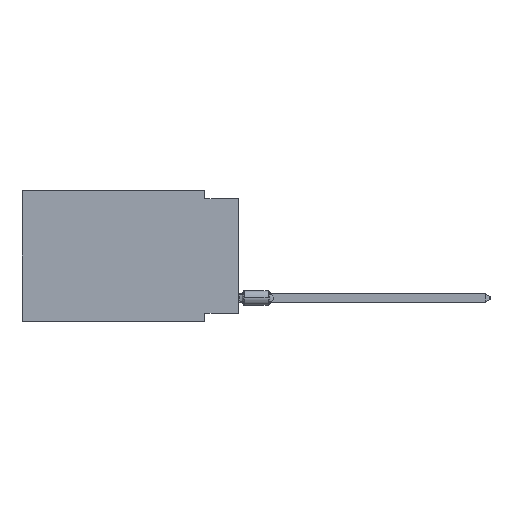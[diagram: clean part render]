
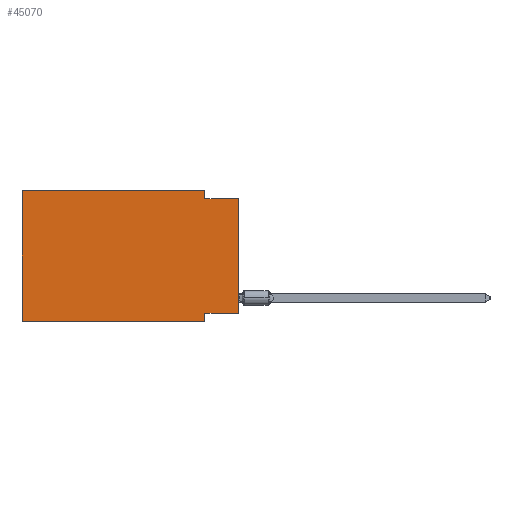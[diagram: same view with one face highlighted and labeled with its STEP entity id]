
A CAD part, left-side view. The second image highlights one B-rep face of the part: STEP entity #45070.
In plain terms, the highlighted planar face has unit normal (-1, 0, 0).
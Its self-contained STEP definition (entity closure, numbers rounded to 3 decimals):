
#275 = DIRECTION ( 'NONE',  ( 0., 0., -1. ) ) ;
#605 = DIRECTION ( 'NONE',  ( 1., 0., 0. ) ) ;
#1259 = DIRECTION ( 'NONE',  ( 0., 0., 1. ) ) ;
#1913 = VERTEX_POINT ( 'NONE', #60325 ) ;
#2238 = EDGE_CURVE ( 'NONE', #56575, #24521, #60573, .T. ) ;
#4235 = LINE ( 'NONE', #50794, #6742 ) ;
#4477 = ORIENTED_EDGE ( 'NONE', *, *, #44353, .F. ) ;
#4780 = VECTOR ( 'NONE', #49890, 1000. ) ;
#6014 = VERTEX_POINT ( 'NONE', #52594 ) ;
#6742 = VECTOR ( 'NONE', #49794, 1000. ) ;
#8410 = CARTESIAN_POINT ( 'NONE',  ( 0., 2.54, -9.906 ) ) ;
#9024 = LINE ( 'NONE', #14387, #4780 ) ;
#10152 = DIRECTION ( 'NONE',  ( 0., 0., -1. ) ) ;
#10315 = PLANE ( 'NONE',  #17072 ) ;
#10420 = EDGE_CURVE ( 'NONE', #21178, #6014, #4235, .T. ) ;
#11224 = VECTOR ( 'NONE', #1259, 1000. ) ;
#11340 = EDGE_CURVE ( 'NONE', #56575, #1913, #37415, .T. ) ;
#12109 = CARTESIAN_POINT ( 'NONE',  ( 0., 16.383, 0. ) ) ;
#12765 = LINE ( 'NONE', #12109, #43569 ) ;
#13588 = VECTOR ( 'NONE', #28830, 1000. ) ;
#14387 = CARTESIAN_POINT ( 'NONE',  ( 0., 16.383, 0. ) ) ;
#15198 = EDGE_CURVE ( 'NONE', #52797, #41607, #12765, .T. ) ;
#15515 = VECTOR ( 'NONE', #45199, 1000. ) ;
#15630 = CARTESIAN_POINT ( 'NONE',  ( 0., 0., -0.635 ) ) ;
#17072 = AXIS2_PLACEMENT_3D ( 'NONE', #35448, #605, #275 ) ;
#17195 = CARTESIAN_POINT ( 'NONE',  ( 0., 2.54, -0.635 ) ) ;
#17649 = CARTESIAN_POINT ( 'NONE',  ( 0., 0., 0. ) ) ;
#18766 = CARTESIAN_POINT ( 'NONE',  ( 0., 16.383, -9.906 ) ) ;
#21178 = VERTEX_POINT ( 'NONE', #18766 ) ;
#23139 = DIRECTION ( 'NONE',  ( 0., -1., 0. ) ) ;
#24521 = VERTEX_POINT ( 'NONE', #55439 ) ;
#24761 = CARTESIAN_POINT ( 'NONE',  ( 0., 0., -9.271 ) ) ;
#26007 = DIRECTION ( 'NONE',  ( 0., -1., 0. ) ) ;
#27126 = VERTEX_POINT ( 'NONE', #17195 ) ;
#28830 = DIRECTION ( 'NONE',  ( 0., 0., -1. ) ) ;
#32337 = ORIENTED_EDGE ( 'NONE', *, *, #40768, .F. ) ;
#35186 = ORIENTED_EDGE ( 'NONE', *, *, #41457, .F. ) ;
#35448 = CARTESIAN_POINT ( 'NONE',  ( 0., 16.383, 0. ) ) ;
#37245 = ORIENTED_EDGE ( 'NONE', *, *, #51117, .F. ) ;
#37415 = LINE ( 'NONE', #17649, #11224 ) ;
#37884 = ORIENTED_EDGE ( 'NONE', *, *, #2238, .F. ) ;
#40768 = EDGE_CURVE ( 'NONE', #21178, #52797, #9024, .T. ) ;
#41457 = EDGE_CURVE ( 'NONE', #27126, #1913, #46446, .T. ) ;
#41607 = VERTEX_POINT ( 'NONE', #59007 ) ;
#42217 = EDGE_LOOP ( 'NONE', ( #54511, #35186, #4477, #50656, #32337, #45189, #37245, #37884 ) ) ;
#42343 = VECTOR ( 'NONE', #26007, 1000. ) ;
#43569 = VECTOR ( 'NONE', #23139, 1000. ) ;
#44353 = EDGE_CURVE ( 'NONE', #41607, #27126, #56025, .T. ) ;
#45070 = ADVANCED_FACE ( 'NONE', ( #46180 ), #10315, .F. ) ;
#45189 = ORIENTED_EDGE ( 'NONE', *, *, #10420, .T. ) ;
#45199 = DIRECTION ( 'NONE',  ( 0., 1., 0. ) ) ;
#45457 = CARTESIAN_POINT ( 'NONE',  ( 0., 16.383, 0. ) ) ;
#46180 = FACE_OUTER_BOUND ( 'NONE', #42217, .T. ) ;
#46446 = LINE ( 'NONE', #15630, #42343 ) ;
#46659 = CARTESIAN_POINT ( 'NONE',  ( 0., 2.54, 0. ) ) ;
#49794 = DIRECTION ( 'NONE',  ( 0., -1., 0. ) ) ;
#49890 = DIRECTION ( 'NONE',  ( 0., 0., 1. ) ) ;
#50656 = ORIENTED_EDGE ( 'NONE', *, *, #15198, .F. ) ;
#50794 = CARTESIAN_POINT ( 'NONE',  ( 0., 16.383, -9.906 ) ) ;
#51117 = EDGE_CURVE ( 'NONE', #24521, #6014, #64323, .T. ) ;
#52594 = CARTESIAN_POINT ( 'NONE',  ( 0., 2.54, -9.906 ) ) ;
#52797 = VERTEX_POINT ( 'NONE', #45457 ) ;
#54226 = VECTOR ( 'NONE', #10152, 1000. ) ;
#54511 = ORIENTED_EDGE ( 'NONE', *, *, #11340, .T. ) ;
#55439 = CARTESIAN_POINT ( 'NONE',  ( 0., 2.54, -9.271 ) ) ;
#56025 = LINE ( 'NONE', #46659, #54226 ) ;
#56575 = VERTEX_POINT ( 'NONE', #62576 ) ;
#59007 = CARTESIAN_POINT ( 'NONE',  ( 0., 2.54, 0. ) ) ;
#60325 = CARTESIAN_POINT ( 'NONE',  ( 0., 0., -0.635 ) ) ;
#60573 = LINE ( 'NONE', #24761, #15515 ) ;
#62576 = CARTESIAN_POINT ( 'NONE',  ( 0., 0., -9.271 ) ) ;
#64323 = LINE ( 'NONE', #8410, #13588 ) ;
